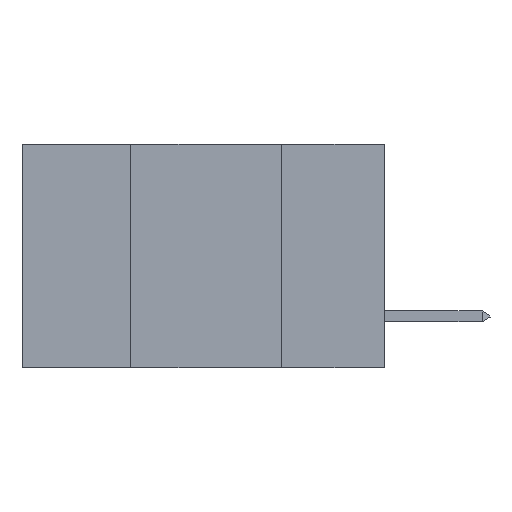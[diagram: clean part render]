
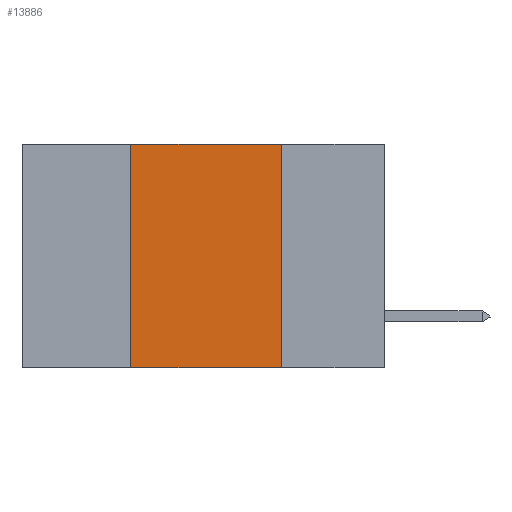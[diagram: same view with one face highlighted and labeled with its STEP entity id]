
A CAD part, left-side view. The second image highlights one B-rep face of the part: STEP entity #13886.
In plain terms, the highlighted planar face has unit normal (-1, 0, 0).
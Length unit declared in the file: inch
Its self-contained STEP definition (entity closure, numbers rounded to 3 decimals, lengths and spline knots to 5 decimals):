
#31 = VERTEX_POINT ( 'NONE', #10724 ) ;
#1017 = FACE_OUTER_BOUND ( 'NONE', #6066, .T. ) ;
#1096 = EDGE_CURVE ( 'NONE', #31, #9141, #1695, .T. ) ;
#1103 = VECTOR ( 'NONE', #12254, 39.37008 ) ;
#1695 = LINE ( 'NONE', #2073, #1103 ) ;
#1784 = ORIENTED_EDGE ( 'NONE', *, *, #1096, .F. ) ;
#2073 = CARTESIAN_POINT ( 'NONE',  ( 0., 0.6, 0. ) ) ;
#2332 = AXIS2_PLACEMENT_3D ( 'NONE', #5990, #7117, #14761 ) ;
#2383 = EDGE_CURVE ( 'NONE', #13762, #31, #15936, .T. ) ;
#3379 = ORIENTED_EDGE ( 'NONE', *, *, #12818, .T. ) ;
#3654 = DIRECTION ( 'NONE',  ( 0., 0., -1. ) ) ;
#5019 = DIRECTION ( 'NONE',  ( 0., 0., 1. ) ) ;
#5374 = ORIENTED_EDGE ( 'NONE', *, *, #5575, .F. ) ;
#5575 = EDGE_CURVE ( 'NONE', #9141, #7728, #7268, .T. ) ;
#5743 = VECTOR ( 'NONE', #6038, 39.37008 ) ;
#5870 = PLANE ( 'NONE',  #2332 ) ;
#5990 = CARTESIAN_POINT ( 'NONE',  ( 0., 0.6, 0. ) ) ;
#6038 = DIRECTION ( 'NONE',  ( 0., -1., 0. ) ) ;
#6066 = EDGE_LOOP ( 'NONE', ( #5374, #1784, #8714, #3379 ) ) ;
#7117 = DIRECTION ( 'NONE',  ( 1., 0., 0. ) ) ;
#7268 = LINE ( 'NONE', #9831, #10251 ) ;
#7728 = VERTEX_POINT ( 'NONE', #15942 ) ;
#8028 = CARTESIAN_POINT ( 'NONE',  ( 0., 0.42, -0.37 ) ) ;
#8623 = VECTOR ( 'NONE', #5019, 39.37008 ) ;
#8714 = ORIENTED_EDGE ( 'NONE', *, *, #2383, .F. ) ;
#9141 = VERTEX_POINT ( 'NONE', #13854 ) ;
#9831 = CARTESIAN_POINT ( 'NONE',  ( 0., 0.17, 0. ) ) ;
#10251 = VECTOR ( 'NONE', #3654, 39.37008 ) ;
#10724 = CARTESIAN_POINT ( 'NONE',  ( 0., 0.42, 0. ) ) ;
#11273 = CARTESIAN_POINT ( 'NONE',  ( 0., 0.6, -0.37 ) ) ;
#12254 = DIRECTION ( 'NONE',  ( 0., -1., 0. ) ) ;
#12444 = CARTESIAN_POINT ( 'NONE',  ( 0., 0.42, 0. ) ) ;
#12818 = EDGE_CURVE ( 'NONE', #13762, #7728, #14727, .T. ) ;
#13762 = VERTEX_POINT ( 'NONE', #8028 ) ;
#13854 = CARTESIAN_POINT ( 'NONE',  ( 0., 0.17, 0. ) ) ;
#13886 = ADVANCED_FACE ( 'NONE', ( #1017 ), #5870, .F. ) ;
#14727 = LINE ( 'NONE', #11273, #5743 ) ;
#14761 = DIRECTION ( 'NONE',  ( 0., 0., -1. ) ) ;
#15936 = LINE ( 'NONE', #12444, #8623 ) ;
#15942 = CARTESIAN_POINT ( 'NONE',  ( 0., 0.17, -0.37 ) ) ;
